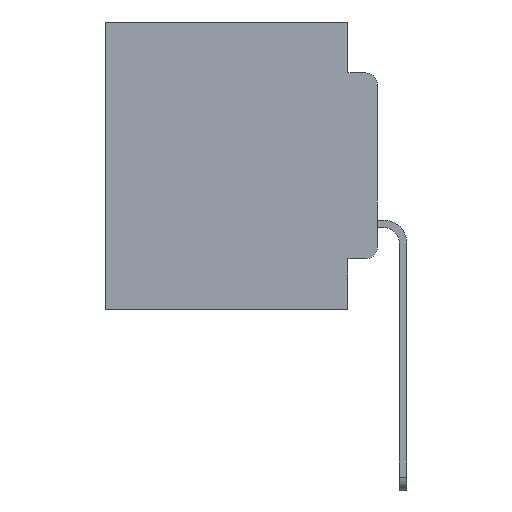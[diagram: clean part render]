
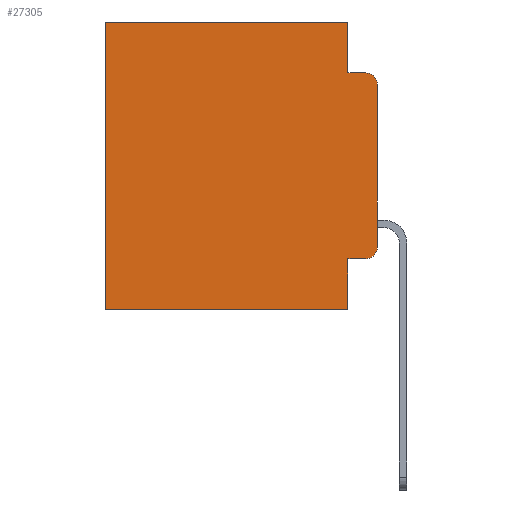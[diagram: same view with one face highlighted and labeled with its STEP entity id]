
A CAD part, left-side view. The second image highlights one B-rep face of the part: STEP entity #27305.
In plain terms, the highlighted planar face has unit normal (-1, 0, 0).
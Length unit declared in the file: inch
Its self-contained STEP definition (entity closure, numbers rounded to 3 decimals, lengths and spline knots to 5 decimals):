
#825 = LINE ( 'NONE', #2474, #12642 ) ;
#862 = EDGE_CURVE ( 'NONE', #12405, #23533, #2067, .T. ) ;
#1239 = EDGE_CURVE ( 'NONE', #13700, #21576, #825, .T. ) ;
#1261 = DIRECTION ( 'NONE',  ( 0., 0., -1. ) ) ;
#1480 = CARTESIAN_POINT ( 'NONE',  ( 0.298, 0.051, -0.4115 ) ) ;
#1549 = DIRECTION ( 'NONE',  ( 0., -1., 0. ) ) ;
#1938 = DIRECTION ( 'NONE',  ( 0., 1., 0. ) ) ;
#2067 = LINE ( 'NONE', #8208, #24788 ) ;
#2299 = EDGE_LOOP ( 'NONE', ( #15037, #26041, #3660, #5234, #12664, #23820, #19605, #25102, #2449, #9482 ) ) ;
#2311 = EDGE_CURVE ( 'NONE', #6512, #16811, #11818, .T. ) ;
#2410 = LINE ( 'NONE', #21371, #25069 ) ;
#2449 = ORIENTED_EDGE ( 'NONE', *, *, #1239, .T. ) ;
#2474 = CARTESIAN_POINT ( 'NONE',  ( 0.298, 0.051, -0.4115 ) ) ;
#2987 = EDGE_CURVE ( 'NONE', #13700, #12405, #7288, .T. ) ;
#3489 = PLANE ( 'NONE',  #25857 ) ;
#3660 = ORIENTED_EDGE ( 'NONE', *, *, #16659, .F. ) ;
#3894 = DIRECTION ( 'NONE',  ( 0., -1., 0. ) ) ;
#4918 = VECTOR ( 'NONE', #1938, 39.37008 ) ;
#5043 = VERTEX_POINT ( 'NONE', #14056 ) ;
#5125 = CARTESIAN_POINT ( 'NONE',  ( 0.298, 0.473, 0. ) ) ;
#5234 = ORIENTED_EDGE ( 'NONE', *, *, #15238, .F. ) ;
#5720 = LINE ( 'NONE', #23110, #16781 ) ;
#5724 = CARTESIAN_POINT ( 'NONE',  ( 0.298, 0.051, 0. ) ) ;
#5751 = DIRECTION ( 'NONE',  ( -1., 0., 0. ) ) ;
#6044 = CIRCLE ( 'NONE', #12218, 0.02 ) ;
#6476 = VERTEX_POINT ( 'NONE', #13743 ) ;
#6512 = VERTEX_POINT ( 'NONE', #20077 ) ;
#6587 = VECTOR ( 'NONE', #12477, 39.37008 ) ;
#7002 = DIRECTION ( 'NONE',  ( 0., 0., -1. ) ) ;
#7288 = LINE ( 'NONE', #5724, #6587 ) ;
#8208 = CARTESIAN_POINT ( 'NONE',  ( 0.298, 0., -0.5 ) ) ;
#8542 = CARTESIAN_POINT ( 'NONE',  ( 0.298, 0.473, 0. ) ) ;
#8936 = CARTESIAN_POINT ( 'NONE',  ( 0.298, 0., 0. ) ) ;
#9273 = EDGE_CURVE ( 'NONE', #26641, #23533, #21081, .T. ) ;
#9482 = ORIENTED_EDGE ( 'NONE', *, *, #22708, .T. ) ;
#10586 = CARTESIAN_POINT ( 'NONE',  ( 0.298, 0.473, -0.5 ) ) ;
#11666 = LINE ( 'NONE', #28033, #4918 ) ;
#11818 = LINE ( 'NONE', #8936, #16920 ) ;
#12218 = AXIS2_PLACEMENT_3D ( 'NONE', #18820, #5751, #20908 ) ;
#12405 = VERTEX_POINT ( 'NONE', #15142 ) ;
#12477 = DIRECTION ( 'NONE',  ( 0., 0., -1. ) ) ;
#12642 = VECTOR ( 'NONE', #1549, 39.37008 ) ;
#12664 = ORIENTED_EDGE ( 'NONE', *, *, #25345, .T. ) ;
#12778 = DIRECTION ( 'NONE',  ( 0., 1., 0. ) ) ;
#13700 = VERTEX_POINT ( 'NONE', #1480 ) ;
#13743 = CARTESIAN_POINT ( 'NONE',  ( 0.298, 0.051, 0. ) ) ;
#14056 = CARTESIAN_POINT ( 'NONE',  ( 0.298, 0.02, -0.0885 ) ) ;
#14497 = CARTESIAN_POINT ( 'NONE',  ( 0.298, 0.051, -0.0885 ) ) ;
#14842 = CARTESIAN_POINT ( 'NONE',  ( 0.298, 0., 0. ) ) ;
#15037 = ORIENTED_EDGE ( 'NONE', *, *, #2311, .F. ) ;
#15142 = CARTESIAN_POINT ( 'NONE',  ( 0.298, 0.051, -0.5 ) ) ;
#15158 = DIRECTION ( 'NONE',  ( -1., 0., 0. ) ) ;
#15238 = EDGE_CURVE ( 'NONE', #6476, #24213, #5720, .T. ) ;
#16659 = EDGE_CURVE ( 'NONE', #24213, #5043, #2410, .T. ) ;
#16781 = VECTOR ( 'NONE', #25167, 39.37008 ) ;
#16811 = VERTEX_POINT ( 'NONE', #17675 ) ;
#16888 = DIRECTION ( 'NONE',  ( 1., 0., 0. ) ) ;
#16920 = VECTOR ( 'NONE', #7002, 39.37008 ) ;
#17675 = CARTESIAN_POINT ( 'NONE',  ( 0.298, 0., -0.3915 ) ) ;
#18037 = EDGE_CURVE ( 'NONE', #6512, #5043, #6044, .T. ) ;
#18820 = CARTESIAN_POINT ( 'NONE',  ( 0.298, 0.02, -0.1085 ) ) ;
#19047 = DIRECTION ( 'NONE',  ( 0., 0., -1. ) ) ;
#19605 = ORIENTED_EDGE ( 'NONE', *, *, #862, .F. ) ;
#20077 = CARTESIAN_POINT ( 'NONE',  ( 0.298, 0., -0.1085 ) ) ;
#20382 = DIRECTION ( 'NONE',  ( 0., 0., -1. ) ) ;
#20628 = CARTESIAN_POINT ( 'NONE',  ( 0.298, 0.02, -0.4115 ) ) ;
#20908 = DIRECTION ( 'NONE',  ( 0., 0., -1. ) ) ;
#21081 = LINE ( 'NONE', #5125, #25893 ) ;
#21371 = CARTESIAN_POINT ( 'NONE',  ( 0.298, 0.051, -0.0885 ) ) ;
#21576 = VERTEX_POINT ( 'NONE', #20628 ) ;
#21832 = CIRCLE ( 'NONE', #24255, 0.02 ) ;
#22708 = EDGE_CURVE ( 'NONE', #21576, #16811, #21832, .T. ) ;
#23110 = CARTESIAN_POINT ( 'NONE',  ( 0.298, 0.051, 0. ) ) ;
#23533 = VERTEX_POINT ( 'NONE', #10586 ) ;
#23820 = ORIENTED_EDGE ( 'NONE', *, *, #9273, .T. ) ;
#24213 = VERTEX_POINT ( 'NONE', #14497 ) ;
#24255 = AXIS2_PLACEMENT_3D ( 'NONE', #27496, #15158, #1261 ) ;
#24721 = FACE_OUTER_BOUND ( 'NONE', #2299, .T. ) ;
#24788 = VECTOR ( 'NONE', #12778, 39.37008 ) ;
#25069 = VECTOR ( 'NONE', #3894, 39.37008 ) ;
#25102 = ORIENTED_EDGE ( 'NONE', *, *, #2987, .F. ) ;
#25167 = DIRECTION ( 'NONE',  ( 0., 0., -1. ) ) ;
#25345 = EDGE_CURVE ( 'NONE', #6476, #26641, #11666, .T. ) ;
#25857 = AXIS2_PLACEMENT_3D ( 'NONE', #14842, #16888, #19047 ) ;
#25893 = VECTOR ( 'NONE', #20382, 39.37008 ) ;
#26041 = ORIENTED_EDGE ( 'NONE', *, *, #18037, .T. ) ;
#26641 = VERTEX_POINT ( 'NONE', #8542 ) ;
#27305 = ADVANCED_FACE ( 'NONE', ( #24721 ), #3489, .F. ) ;
#27496 = CARTESIAN_POINT ( 'NONE',  ( 0.298, 0.02, -0.3915 ) ) ;
#28033 = CARTESIAN_POINT ( 'NONE',  ( 0.298, 0., 0. ) ) ;
